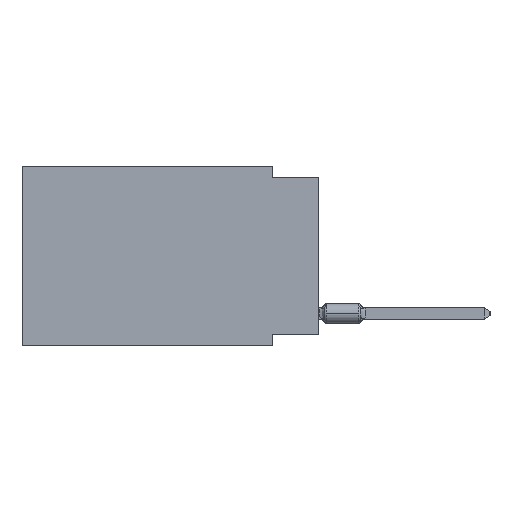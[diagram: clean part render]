
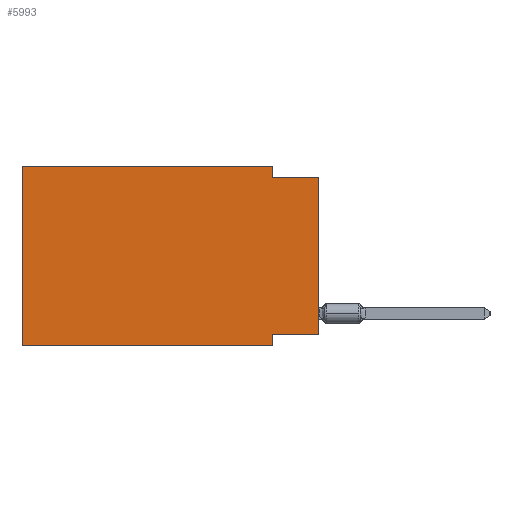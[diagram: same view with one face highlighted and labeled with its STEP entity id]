
A CAD part, left-side view. The second image highlights one B-rep face of the part: STEP entity #5993.
In plain terms, the highlighted planar face has unit normal (-1, 0, 0).
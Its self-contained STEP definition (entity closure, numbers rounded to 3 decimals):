
#1507 = CARTESIAN_POINT ( 'NONE',  ( 0., 2.54, -9.906 ) ) ;
#2765 = VECTOR ( 'NONE', #27831, 1000. ) ;
#3161 = EDGE_LOOP ( 'NONE', ( #31174, #34762, #25627, #23562, #23986, #13399, #20806, #15239 ) ) ;
#3181 = LINE ( 'NONE', #11930, #2765 ) ;
#4480 = VECTOR ( 'NONE', #35905, 1000. ) ;
#4500 = LINE ( 'NONE', #35332, #15798 ) ;
#5081 = EDGE_CURVE ( 'NONE', #6106, #12955, #31276, .T. ) ;
#5402 = CARTESIAN_POINT ( 'NONE',  ( 0., 2.54, -9.906 ) ) ;
#5993 = ADVANCED_FACE ( 'NONE', ( #14686 ), #12312, .F. ) ;
#6106 = VERTEX_POINT ( 'NONE', #7393 ) ;
#6206 = VECTOR ( 'NONE', #21628, 1000. ) ;
#6364 = VECTOR ( 'NONE', #19923, 1000. ) ;
#7393 = CARTESIAN_POINT ( 'NONE',  ( 0., 16.383, -9.906 ) ) ;
#7460 = VERTEX_POINT ( 'NONE', #25065 ) ;
#9169 = LINE ( 'NONE', #17539, #6364 ) ;
#9893 = CARTESIAN_POINT ( 'NONE',  ( 0., 2.54, -9.271 ) ) ;
#10581 = AXIS2_PLACEMENT_3D ( 'NONE', #29114, #12675, #31490 ) ;
#11918 = CARTESIAN_POINT ( 'NONE',  ( 0., 16.383, 0. ) ) ;
#11930 = CARTESIAN_POINT ( 'NONE',  ( 0., 0., 0. ) ) ;
#12312 = PLANE ( 'NONE',  #10581 ) ;
#12675 = DIRECTION ( 'NONE',  ( 1., 0., 0. ) ) ;
#12955 = VERTEX_POINT ( 'NONE', #18440 ) ;
#13355 = VECTOR ( 'NONE', #27298, 1000. ) ;
#13399 = ORIENTED_EDGE ( 'NONE', *, *, #23741, .T. ) ;
#14686 = FACE_OUTER_BOUND ( 'NONE', #3161, .T. ) ;
#15239 = ORIENTED_EDGE ( 'NONE', *, *, #22923, .F. ) ;
#15393 = VECTOR ( 'NONE', #30326, 1000. ) ;
#15798 = VECTOR ( 'NONE', #29695, 1000. ) ;
#16049 = CARTESIAN_POINT ( 'NONE',  ( 0., 2.54, -0.635 ) ) ;
#16130 = CARTESIAN_POINT ( 'NONE',  ( 0., 0., -9.271 ) ) ;
#16315 = LINE ( 'NONE', #16130, #6206 ) ;
#16325 = EDGE_CURVE ( 'NONE', #27163, #7460, #25010, .T. ) ;
#16362 = LINE ( 'NONE', #27512, #4480 ) ;
#17539 = CARTESIAN_POINT ( 'NONE',  ( 0., 2.54, 0. ) ) ;
#18440 = CARTESIAN_POINT ( 'NONE',  ( 0., 16.383, 0. ) ) ;
#18896 = LINE ( 'NONE', #5402, #13355 ) ;
#19923 = DIRECTION ( 'NONE',  ( 0., 0., -1. ) ) ;
#20806 = ORIENTED_EDGE ( 'NONE', *, *, #27659, .F. ) ;
#20809 = VERTEX_POINT ( 'NONE', #28411 ) ;
#21628 = DIRECTION ( 'NONE',  ( 0., 1., 0. ) ) ;
#22862 = DIRECTION ( 'NONE',  ( 0., 0., 1. ) ) ;
#22923 = EDGE_CURVE ( 'NONE', #20809, #28380, #16315, .T. ) ;
#23562 = ORIENTED_EDGE ( 'NONE', *, *, #29700, .F. ) ;
#23741 = EDGE_CURVE ( 'NONE', #6106, #31674, #16362, .T. ) ;
#23986 = ORIENTED_EDGE ( 'NONE', *, *, #5081, .F. ) ;
#24242 = EDGE_CURVE ( 'NONE', #20809, #7460, #3181, .T. ) ;
#25010 = LINE ( 'NONE', #35616, #15393 ) ;
#25065 = CARTESIAN_POINT ( 'NONE',  ( 0., 0., -0.635 ) ) ;
#25627 = ORIENTED_EDGE ( 'NONE', *, *, #34309, .F. ) ;
#25642 = VERTEX_POINT ( 'NONE', #31715 ) ;
#27163 = VERTEX_POINT ( 'NONE', #16049 ) ;
#27298 = DIRECTION ( 'NONE',  ( 0., 0., -1. ) ) ;
#27512 = CARTESIAN_POINT ( 'NONE',  ( 0., 16.383, -9.906 ) ) ;
#27659 = EDGE_CURVE ( 'NONE', #28380, #31674, #18896, .T. ) ;
#27831 = DIRECTION ( 'NONE',  ( 0., 0., 1. ) ) ;
#28380 = VERTEX_POINT ( 'NONE', #9893 ) ;
#28411 = CARTESIAN_POINT ( 'NONE',  ( 0., 0., -9.271 ) ) ;
#29114 = CARTESIAN_POINT ( 'NONE',  ( 0., 16.383, 0. ) ) ;
#29695 = DIRECTION ( 'NONE',  ( 0., -1., 0. ) ) ;
#29700 = EDGE_CURVE ( 'NONE', #12955, #25642, #4500, .T. ) ;
#30326 = DIRECTION ( 'NONE',  ( 0., -1., 0. ) ) ;
#31174 = ORIENTED_EDGE ( 'NONE', *, *, #24242, .T. ) ;
#31276 = LINE ( 'NONE', #11918, #35234 ) ;
#31490 = DIRECTION ( 'NONE',  ( 0., 0., -1. ) ) ;
#31674 = VERTEX_POINT ( 'NONE', #1507 ) ;
#31715 = CARTESIAN_POINT ( 'NONE',  ( 0., 2.54, 0. ) ) ;
#34309 = EDGE_CURVE ( 'NONE', #25642, #27163, #9169, .T. ) ;
#34762 = ORIENTED_EDGE ( 'NONE', *, *, #16325, .F. ) ;
#35234 = VECTOR ( 'NONE', #22862, 1000. ) ;
#35332 = CARTESIAN_POINT ( 'NONE',  ( 0., 16.383, 0. ) ) ;
#35616 = CARTESIAN_POINT ( 'NONE',  ( 0., 0., -0.635 ) ) ;
#35905 = DIRECTION ( 'NONE',  ( 0., -1., 0. ) ) ;
